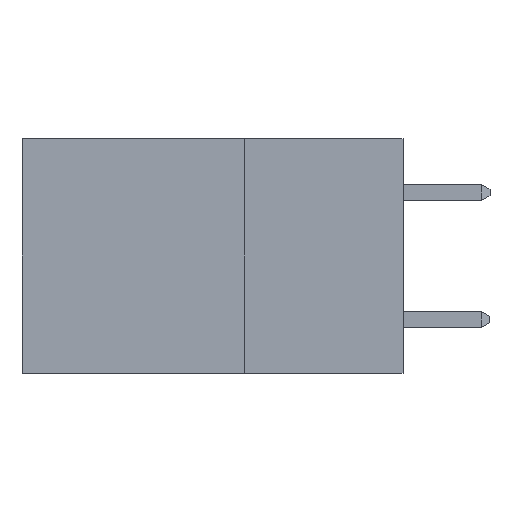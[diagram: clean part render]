
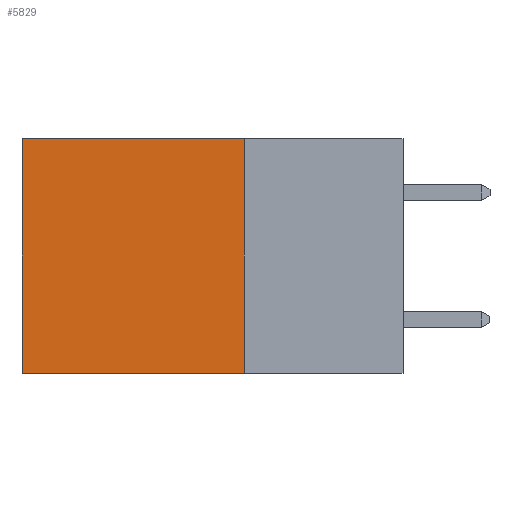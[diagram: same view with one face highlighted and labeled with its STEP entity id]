
A CAD part, left-side view. The second image highlights one B-rep face of the part: STEP entity #5829.
In plain terms, the highlighted planar face has unit normal (-1, 0, 0).
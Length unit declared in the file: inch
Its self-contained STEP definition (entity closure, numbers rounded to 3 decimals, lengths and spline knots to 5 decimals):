
#55 = LINE ( 'NONE', #106, #4356 ) ;
#63 = DIRECTION ( 'NONE',  ( 0., 0., -1. ) ) ;
#106 = CARTESIAN_POINT ( 'NONE',  ( 0.2875, 0.25, -0.37 ) ) ;
#177 = DIRECTION ( 'NONE',  ( 0., 0., -1. ) ) ;
#505 = EDGE_CURVE ( 'NONE', #5603, #4939, #4329, .T. ) ;
#780 = VERTEX_POINT ( 'NONE', #6291 ) ;
#1244 = CARTESIAN_POINT ( 'NONE',  ( 0.2875, 0.25, 0. ) ) ;
#1600 = EDGE_LOOP ( 'NONE', ( #3968, #4360, #3768, #3902 ) ) ;
#1756 = EDGE_CURVE ( 'NONE', #780, #5603, #4379, .T. ) ;
#2477 = VERTEX_POINT ( 'NONE', #2646 ) ;
#2646 = CARTESIAN_POINT ( 'NONE',  ( 0.2875, 0.25, -0.37 ) ) ;
#2963 = VECTOR ( 'NONE', #7253, 39.37008 ) ;
#3297 = VECTOR ( 'NONE', #7095, 39.37008 ) ;
#3645 = DIRECTION ( 'NONE',  ( 1., 0., 0. ) ) ;
#3768 = ORIENTED_EDGE ( 'NONE', *, *, #8771, .F. ) ;
#3902 = ORIENTED_EDGE ( 'NONE', *, *, #1756, .T. ) ;
#3968 = ORIENTED_EDGE ( 'NONE', *, *, #505, .T. ) ;
#4150 = VECTOR ( 'NONE', #63, 39.37008 ) ;
#4227 = LINE ( 'NONE', #1244, #3297 ) ;
#4329 = LINE ( 'NONE', #8715, #4150 ) ;
#4356 = VECTOR ( 'NONE', #6490, 39.37008 ) ;
#4360 = ORIENTED_EDGE ( 'NONE', *, *, #8939, .F. ) ;
#4379 = LINE ( 'NONE', #4469, #2963 ) ;
#4469 = CARTESIAN_POINT ( 'NONE',  ( 0.2875, 0.25, 0. ) ) ;
#4939 = VERTEX_POINT ( 'NONE', #8801 ) ;
#5235 = CARTESIAN_POINT ( 'NONE',  ( 0.2875, 0.25, 0. ) ) ;
#5603 = VERTEX_POINT ( 'NONE', #7734 ) ;
#5829 = ADVANCED_FACE ( 'NONE', ( #6653 ), #7311, .F. ) ;
#6291 = CARTESIAN_POINT ( 'NONE',  ( 0.2875, 0.25, 0. ) ) ;
#6490 = DIRECTION ( 'NONE',  ( 0., 1., 0. ) ) ;
#6653 = FACE_OUTER_BOUND ( 'NONE', #1600, .T. ) ;
#7095 = DIRECTION ( 'NONE',  ( 0., 0., -1. ) ) ;
#7253 = DIRECTION ( 'NONE',  ( 0., 1., 0. ) ) ;
#7311 = PLANE ( 'NONE',  #7761 ) ;
#7734 = CARTESIAN_POINT ( 'NONE',  ( 0.2875, 0.6, 0. ) ) ;
#7761 = AXIS2_PLACEMENT_3D ( 'NONE', #5235, #3645, #177 ) ;
#8715 = CARTESIAN_POINT ( 'NONE',  ( 0.2875, 0.6, 0. ) ) ;
#8771 = EDGE_CURVE ( 'NONE', #780, #2477, #4227, .T. ) ;
#8801 = CARTESIAN_POINT ( 'NONE',  ( 0.2875, 0.6, -0.37 ) ) ;
#8939 = EDGE_CURVE ( 'NONE', #2477, #4939, #55, .T. ) ;
